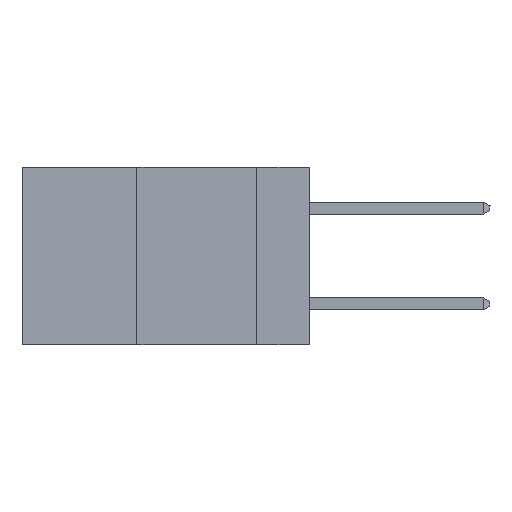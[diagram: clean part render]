
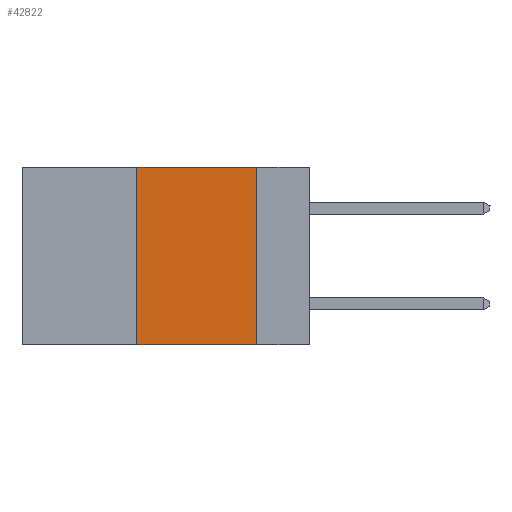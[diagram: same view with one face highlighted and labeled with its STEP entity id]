
A CAD part, left-side view. The second image highlights one B-rep face of the part: STEP entity #42822.
In plain terms, the highlighted planar face has unit normal (-1, 0, 0).
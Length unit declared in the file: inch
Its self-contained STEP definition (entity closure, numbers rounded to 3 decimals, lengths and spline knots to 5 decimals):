
#4536 = PLANE ( 'NONE',  #26797 ) ;
#4576 = DIRECTION ( 'NONE',  ( 0., -1., 0. ) ) ;
#4789 = CARTESIAN_POINT ( 'NONE',  ( 0., 0.6, -0.37 ) ) ;
#6324 = DIRECTION ( 'NONE',  ( 0., 0., 1. ) ) ;
#10432 = DIRECTION ( 'NONE',  ( 0., -1., 0. ) ) ;
#11361 = EDGE_CURVE ( 'NONE', #34225, #27223, #45130, .T. ) ;
#11492 = ORIENTED_EDGE ( 'NONE', *, *, #23348, .F. ) ;
#12468 = VERTEX_POINT ( 'NONE', #17959 ) ;
#13309 = FACE_OUTER_BOUND ( 'NONE', #18506, .T. ) ;
#13869 = CARTESIAN_POINT ( 'NONE',  ( 0., 0.6, 0. ) ) ;
#14488 = CARTESIAN_POINT ( 'NONE',  ( 0., 0.36, -0.37 ) ) ;
#15323 = ORIENTED_EDGE ( 'NONE', *, *, #11361, .T. ) ;
#17959 = CARTESIAN_POINT ( 'NONE',  ( 0., 0.11, 0. ) ) ;
#18324 = DIRECTION ( 'NONE',  ( 0., 0., -1. ) ) ;
#18506 = EDGE_LOOP ( 'NONE', ( #23431, #11492, #27636, #15323 ) ) ;
#19004 = CARTESIAN_POINT ( 'NONE',  ( 0., 0.6, 0. ) ) ;
#19281 = CARTESIAN_POINT ( 'NONE',  ( 0., 0.11, -0.37 ) ) ;
#19834 = CARTESIAN_POINT ( 'NONE',  ( 0., 0.36, 0. ) ) ;
#22545 = DIRECTION ( 'NONE',  ( 0., 0., -1. ) ) ;
#23348 = EDGE_CURVE ( 'NONE', #42299, #12468, #37944, .T. ) ;
#23431 = ORIENTED_EDGE ( 'NONE', *, *, #39478, .F. ) ;
#24106 = CARTESIAN_POINT ( 'NONE',  ( 0., 0.36, 0. ) ) ;
#26797 = AXIS2_PLACEMENT_3D ( 'NONE', #19004, #43250, #22545 ) ;
#27223 = VERTEX_POINT ( 'NONE', #19281 ) ;
#27636 = ORIENTED_EDGE ( 'NONE', *, *, #39932, .F. ) ;
#34166 = VECTOR ( 'NONE', #6324, 39.37008 ) ;
#34225 = VERTEX_POINT ( 'NONE', #14488 ) ;
#34412 = LINE ( 'NONE', #24106, #34166 ) ;
#35747 = CARTESIAN_POINT ( 'NONE',  ( 0., 0.11, 0. ) ) ;
#37283 = VECTOR ( 'NONE', #18324, 39.37008 ) ;
#37382 = LINE ( 'NONE', #35747, #37283 ) ;
#37936 = VECTOR ( 'NONE', #10432, 39.37008 ) ;
#37944 = LINE ( 'NONE', #13869, #37936 ) ;
#39478 = EDGE_CURVE ( 'NONE', #12468, #27223, #37382, .T. ) ;
#39932 = EDGE_CURVE ( 'NONE', #34225, #42299, #34412, .T. ) ;
#42299 = VERTEX_POINT ( 'NONE', #19834 ) ;
#42822 = ADVANCED_FACE ( 'NONE', ( #13309 ), #4536, .F. ) ;
#43250 = DIRECTION ( 'NONE',  ( 1., 0., 0. ) ) ;
#45130 = LINE ( 'NONE', #4789, #45382 ) ;
#45382 = VECTOR ( 'NONE', #4576, 39.37008 ) ;
